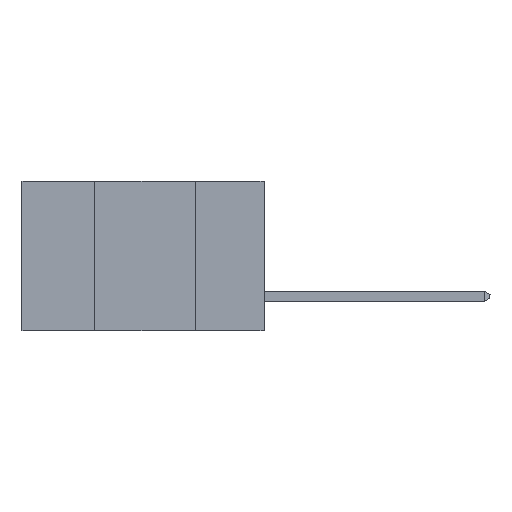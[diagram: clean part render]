
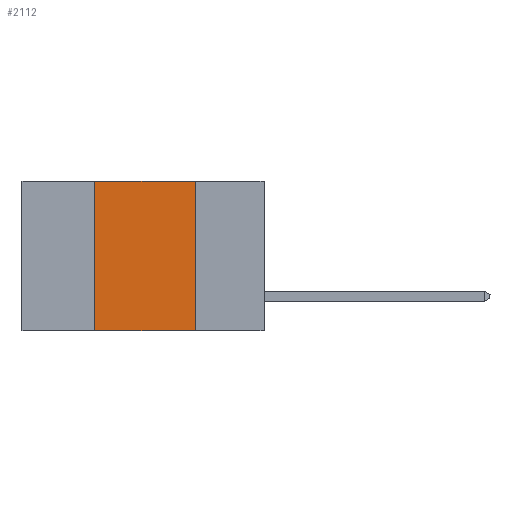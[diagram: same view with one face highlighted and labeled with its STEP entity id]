
A CAD part, left-side view. The second image highlights one B-rep face of the part: STEP entity #2112.
In plain terms, the highlighted planar face has unit normal (-1, 0, 0).
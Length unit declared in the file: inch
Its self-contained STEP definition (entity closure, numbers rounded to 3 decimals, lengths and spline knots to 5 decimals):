
#403 = VECTOR ( 'NONE', #5882, 39.37008 ) ;
#588 = VERTEX_POINT ( 'NONE', #11774 ) ;
#1462 = CARTESIAN_POINT ( 'NONE',  ( 0., 0.6, -0.37 ) ) ;
#2112 = ADVANCED_FACE ( 'NONE', ( #16009 ), #11332, .F. ) ;
#2860 = EDGE_LOOP ( 'NONE', ( #12326, #9711, #12103, #8520 ) ) ;
#3686 = LINE ( 'NONE', #14323, #8978 ) ;
#3856 = DIRECTION ( 'NONE',  ( 1., 0., 0. ) ) ;
#4275 = EDGE_CURVE ( 'NONE', #18436, #8040, #8546, .T. ) ;
#4293 = LINE ( 'NONE', #14841, #403 ) ;
#5882 = DIRECTION ( 'NONE',  ( 0., 0., -1. ) ) ;
#5949 = DIRECTION ( 'NONE',  ( 0., 0., 1. ) ) ;
#6775 = DIRECTION ( 'NONE',  ( 0., 0., -1. ) ) ;
#7031 = CARTESIAN_POINT ( 'NONE',  ( 0., 0.6, 0. ) ) ;
#8037 = CARTESIAN_POINT ( 'NONE',  ( 0., 0.42, 0. ) ) ;
#8040 = VERTEX_POINT ( 'NONE', #8037 ) ;
#8520 = ORIENTED_EDGE ( 'NONE', *, *, #18657, .T. ) ;
#8546 = LINE ( 'NONE', #11913, #10642 ) ;
#8690 = VERTEX_POINT ( 'NONE', #18027 ) ;
#8739 = AXIS2_PLACEMENT_3D ( 'NONE', #7031, #3856, #6775 ) ;
#8859 = DIRECTION ( 'NONE',  ( 0., -1., 0. ) ) ;
#8978 = VECTOR ( 'NONE', #17335, 39.37008 ) ;
#9711 = ORIENTED_EDGE ( 'NONE', *, *, #18998, .F. ) ;
#10334 = CARTESIAN_POINT ( 'NONE',  ( 0., 0.42, -0.37 ) ) ;
#10642 = VECTOR ( 'NONE', #5949, 39.37008 ) ;
#11321 = LINE ( 'NONE', #1462, #13900 ) ;
#11332 = PLANE ( 'NONE',  #8739 ) ;
#11774 = CARTESIAN_POINT ( 'NONE',  ( 0., 0.17, -0.37 ) ) ;
#11795 = EDGE_CURVE ( 'NONE', #8690, #588, #4293, .T. ) ;
#11913 = CARTESIAN_POINT ( 'NONE',  ( 0., 0.42, 0. ) ) ;
#12103 = ORIENTED_EDGE ( 'NONE', *, *, #4275, .F. ) ;
#12326 = ORIENTED_EDGE ( 'NONE', *, *, #11795, .F. ) ;
#13900 = VECTOR ( 'NONE', #8859, 39.37008 ) ;
#14323 = CARTESIAN_POINT ( 'NONE',  ( 0., 0.6, 0. ) ) ;
#14841 = CARTESIAN_POINT ( 'NONE',  ( 0., 0.17, 0. ) ) ;
#16009 = FACE_OUTER_BOUND ( 'NONE', #2860, .T. ) ;
#17335 = DIRECTION ( 'NONE',  ( 0., -1., 0. ) ) ;
#18027 = CARTESIAN_POINT ( 'NONE',  ( 0., 0.17, 0. ) ) ;
#18436 = VERTEX_POINT ( 'NONE', #10334 ) ;
#18657 = EDGE_CURVE ( 'NONE', #18436, #588, #11321, .T. ) ;
#18998 = EDGE_CURVE ( 'NONE', #8040, #8690, #3686, .T. ) ;
